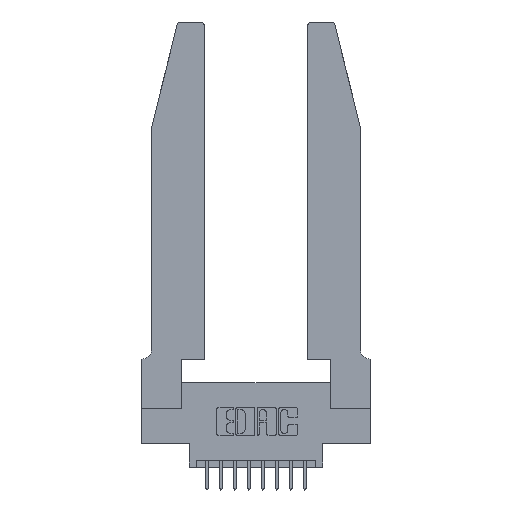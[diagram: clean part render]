
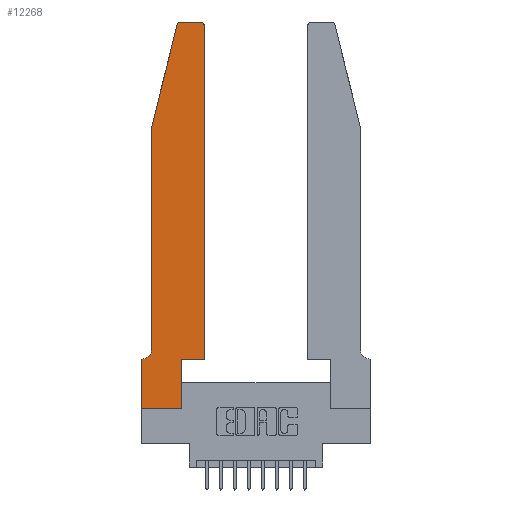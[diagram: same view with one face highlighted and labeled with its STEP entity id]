
A CAD part, top view. The second image highlights one B-rep face of the part: STEP entity #12268.
In plain terms, the highlighted planar face has unit normal (0, 0, 1).
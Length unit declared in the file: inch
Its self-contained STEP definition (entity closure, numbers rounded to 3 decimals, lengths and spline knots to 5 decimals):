
#65 = DIRECTION ( 'NONE',  ( 1., 0., 0. ) ) ;
#135 = VERTEX_POINT ( 'NONE', #9654 ) ;
#272 = CARTESIAN_POINT ( 'NONE',  ( 0.0755, 2., 0.37 ) ) ;
#417 = ORIENTED_EDGE ( 'NONE', *, *, #6303, .T. ) ;
#441 = EDGE_CURVE ( 'NONE', #9025, #10614, #2228, .T. ) ;
#521 = LINE ( 'NONE', #10985, #9922 ) ;
#666 = CARTESIAN_POINT ( 'NONE',  ( 0.284, 2.75, 0.37 ) ) ;
#870 = AXIS2_PLACEMENT_3D ( 'NONE', #2080, #10615, #3317 ) ;
#936 = ORIENTED_EDGE ( 'NONE', *, *, #7987, .T. ) ;
#1139 = AXIS2_PLACEMENT_3D ( 'NONE', #5699, #6950, #15457 ) ;
#1272 = LINE ( 'NONE', #2439, #6628 ) ;
#1345 = ORIENTED_EDGE ( 'NONE', *, *, #4263, .T. ) ;
#1545 = CARTESIAN_POINT ( 'NONE',  ( 0.4505, 0.35, 0.37 ) ) ;
#1622 = LINE ( 'NONE', #6873, #4900 ) ;
#1811 = ORIENTED_EDGE ( 'NONE', *, *, #12740, .T. ) ;
#1819 = VECTOR ( 'NONE', #5220, 39.37008 ) ;
#1833 = LINE ( 'NONE', #2369, #4731 ) ;
#1842 = LINE ( 'NONE', #1545, #8378 ) ;
#2018 = CARTESIAN_POINT ( 'NONE',  ( 0.4505, 0.35, 0.37 ) ) ;
#2080 = CARTESIAN_POINT ( 'NONE',  ( 0.284, 2.72, 0.37 ) ) ;
#2228 = LINE ( 'NONE', #272, #1819 ) ;
#2327 = VERTEX_POINT ( 'NONE', #14522 ) ;
#2369 = CARTESIAN_POINT ( 'NONE',  ( 0.2865, 0.35, 0.37 ) ) ;
#2438 = DIRECTION ( 'NONE',  ( 1., 0., 0. ) ) ;
#2439 = CARTESIAN_POINT ( 'NONE',  ( 0., 0., 0.37 ) ) ;
#2651 = VECTOR ( 'NONE', #9872, 39.37008 ) ;
#2689 = VERTEX_POINT ( 'NONE', #666 ) ;
#2867 = VERTEX_POINT ( 'NONE', #10470 ) ;
#3019 = LINE ( 'NONE', #14705, #9153 ) ;
#3317 = DIRECTION ( 'NONE',  ( 1., 0., 0. ) ) ;
#3345 = EDGE_CURVE ( 'NONE', #7887, #12583, #11640, .T. ) ;
#3458 = CARTESIAN_POINT ( 'NONE',  ( 0.4205, 2.75, 0.37 ) ) ;
#3969 = VECTOR ( 'NONE', #6219, 39.37008 ) ;
#4119 = AXIS2_PLACEMENT_3D ( 'NONE', #12314, #5015, #13552 ) ;
#4165 = CARTESIAN_POINT ( 'NONE',  ( 0.4205, 2.72, 0.37 ) ) ;
#4263 = EDGE_CURVE ( 'NONE', #2327, #135, #521, .T. ) ;
#4310 = EDGE_CURVE ( 'NONE', #9794, #6277, #3019, .T. ) ;
#4311 = EDGE_CURVE ( 'NONE', #2867, #5221, #12398, .T. ) ;
#4482 = PLANE ( 'NONE',  #1139 ) ;
#4731 = VECTOR ( 'NONE', #4841, 39.37008 ) ;
#4841 = DIRECTION ( 'NONE',  ( 0., 1., 0. ) ) ;
#4900 = VECTOR ( 'NONE', #14178, 39.37008 ) ;
#5015 = DIRECTION ( 'NONE',  ( 0., 0., -1. ) ) ;
#5220 = DIRECTION ( 'NONE',  ( -0.239, -0.971, 0. ) ) ;
#5221 = VERTEX_POINT ( 'NONE', #10260 ) ;
#5396 = DIRECTION ( 'NONE',  ( 1., 0., 0. ) ) ;
#5471 = ORIENTED_EDGE ( 'NONE', *, *, #441, .T. ) ;
#5699 = CARTESIAN_POINT ( 'NONE',  ( 0., 0.35, 0.37 ) ) ;
#6044 = EDGE_CURVE ( 'NONE', #6277, #7887, #1842, .T. ) ;
#6219 = DIRECTION ( 'NONE',  ( -1., 0., 0. ) ) ;
#6277 = VERTEX_POINT ( 'NONE', #2018 ) ;
#6303 = EDGE_CURVE ( 'NONE', #2689, #9025, #8576, .T. ) ;
#6628 = VECTOR ( 'NONE', #8551, 39.37008 ) ;
#6873 = CARTESIAN_POINT ( 'NONE',  ( 0.0755, 2., 0.37 ) ) ;
#6950 = DIRECTION ( 'NONE',  ( 0., 0., 1. ) ) ;
#7277 = FACE_OUTER_BOUND ( 'NONE', #12445, .T. ) ;
#7555 = ORIENTED_EDGE ( 'NONE', *, *, #6044, .T. ) ;
#7887 = VERTEX_POINT ( 'NONE', #11545 ) ;
#7987 = EDGE_CURVE ( 'NONE', #10614, #13149, #1622, .T. ) ;
#8378 = VECTOR ( 'NONE', #11327, 39.37008 ) ;
#8551 = DIRECTION ( 'NONE',  ( 0., -1., 0. ) ) ;
#8576 = CIRCLE ( 'NONE', #870, 0.03 ) ;
#8660 = CARTESIAN_POINT ( 'NONE',  ( 0.0755, 0.35, 0.37 ) ) ;
#9025 = VERTEX_POINT ( 'NONE', #11324 ) ;
#9111 = ORIENTED_EDGE ( 'NONE', *, *, #13444, .T. ) ;
#9153 = VECTOR ( 'NONE', #65, 39.37008 ) ;
#9654 = CARTESIAN_POINT ( 'NONE',  ( 0.2865, 0., 0.37 ) ) ;
#9794 = VERTEX_POINT ( 'NONE', #10864 ) ;
#9853 = CARTESIAN_POINT ( 'NONE',  ( 0.2605, 2.75, 0.37 ) ) ;
#9872 = DIRECTION ( 'NONE',  ( -1., 0., 0. ) ) ;
#9922 = VECTOR ( 'NONE', #2438, 39.37008 ) ;
#10260 = CARTESIAN_POINT ( 'NONE',  ( 0., 0.35, 0.37 ) ) ;
#10470 = CARTESIAN_POINT ( 'NONE',  ( 0.0055, 0.35, 0.37 ) ) ;
#10614 = VERTEX_POINT ( 'NONE', #15143 ) ;
#10615 = DIRECTION ( 'NONE',  ( 0., 0., 1. ) ) ;
#10864 = CARTESIAN_POINT ( 'NONE',  ( 0.2865, 0.35, 0.37 ) ) ;
#10933 = ORIENTED_EDGE ( 'NONE', *, *, #4310, .T. ) ;
#10985 = CARTESIAN_POINT ( 'NONE',  ( 0., 0., 0.37 ) ) ;
#11324 = CARTESIAN_POINT ( 'NONE',  ( 0.25487, 2.72718, 0.37 ) ) ;
#11327 = DIRECTION ( 'NONE',  ( 0., 1., 0. ) ) ;
#11545 = CARTESIAN_POINT ( 'NONE',  ( 0.4505, 2.72, 0.37 ) ) ;
#11640 = CIRCLE ( 'NONE', #15416, 0.03 ) ;
#12268 = ADVANCED_FACE ( 'NONE', ( #7277 ), #4482, .T. ) ;
#12314 = CARTESIAN_POINT ( 'NONE',  ( 0.0055, 0.42, 0.37 ) ) ;
#12390 = CIRCLE ( 'NONE', #4119, 0.07 ) ;
#12398 = LINE ( 'NONE', #8660, #2651 ) ;
#12445 = EDGE_LOOP ( 'NONE', ( #9111, #417, #5471, #936, #1811, #13562, #14555, #1345, #14930, #10933, #7555, #14355 ) ) ;
#12583 = VERTEX_POINT ( 'NONE', #3458 ) ;
#12702 = DIRECTION ( 'NONE',  ( 0., 0., 1. ) ) ;
#12740 = EDGE_CURVE ( 'NONE', #13149, #2867, #12390, .T. ) ;
#13149 = VERTEX_POINT ( 'NONE', #15381 ) ;
#13368 = EDGE_CURVE ( 'NONE', #135, #9794, #1833, .T. ) ;
#13444 = EDGE_CURVE ( 'NONE', #12583, #2689, #13702, .T. ) ;
#13552 = DIRECTION ( 'NONE',  ( -1., 0., 0. ) ) ;
#13562 = ORIENTED_EDGE ( 'NONE', *, *, #4311, .T. ) ;
#13702 = LINE ( 'NONE', #9853, #3969 ) ;
#14178 = DIRECTION ( 'NONE',  ( 0., -1., 0. ) ) ;
#14355 = ORIENTED_EDGE ( 'NONE', *, *, #3345, .T. ) ;
#14442 = EDGE_CURVE ( 'NONE', #5221, #2327, #1272, .T. ) ;
#14522 = CARTESIAN_POINT ( 'NONE',  ( 0., 0., 0.37 ) ) ;
#14555 = ORIENTED_EDGE ( 'NONE', *, *, #14442, .T. ) ;
#14705 = CARTESIAN_POINT ( 'NONE',  ( 0.4505, 0.35, 0.37 ) ) ;
#14930 = ORIENTED_EDGE ( 'NONE', *, *, #13368, .T. ) ;
#15143 = CARTESIAN_POINT ( 'NONE',  ( 0.0755, 2., 0.37 ) ) ;
#15381 = CARTESIAN_POINT ( 'NONE',  ( 0.0755, 0.42, 0.37 ) ) ;
#15416 = AXIS2_PLACEMENT_3D ( 'NONE', #4165, #12702, #5396 ) ;
#15457 = DIRECTION ( 'NONE',  ( 1., 0., 0. ) ) ;
